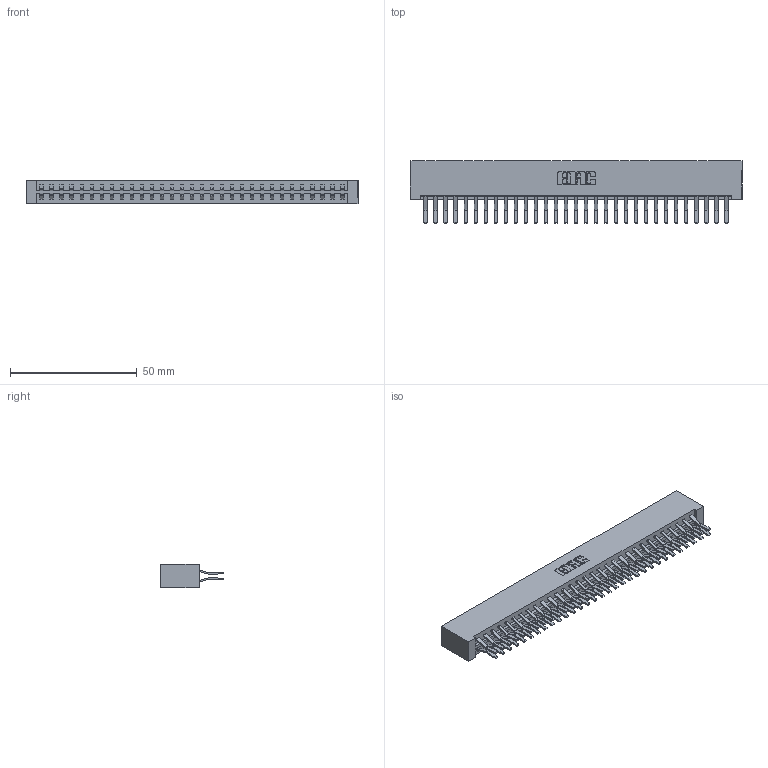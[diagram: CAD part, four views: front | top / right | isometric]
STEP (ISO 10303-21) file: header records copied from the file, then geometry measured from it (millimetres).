
FILE_DESCRIPTION (( 'STEP AP203' ), '1' );
FILE_NAME ('833-062-560-201.STEP', '2020-06-05T06:26:46', ( '' ), ( '' ), 'SwSTEP 2.0', 'SolidWorks 2020', '' );
FILE_SCHEMA (( 'CONFIG_CONTROL_DESIGN' ));
Length unit declared in the file: inch
Products named in the file (3): 833-062-560-201; 833 Part_Lugless; 345-292-001_560 Tail
Assembly tree (63 placements, depth 2):
  833-062-560-201
    833 Part_Lugless
    345-292-001_560 Tail  x62
Bounding box: 131.09 x 24.78 x 9.4 mm (x, y, z)
Volume: 14319.2 mm3; surface area: 17994.3 mm2
Topology: 63 solids, 63 shells, 3454 faces, 10269 edges, 6762 vertices
Faces by surface type: plane 2298, cylinder 1156
Entity records: 21177 total; most frequent: CARTESIAN_POINT 3522, ORIENTED_EDGE 3458, DIRECTION 3025, EDGE_CURVE 1729, LINE 1605, VECTOR 1605, VERTEX_POINT 1150, AXIS2_PLACEMENT_3D 710
